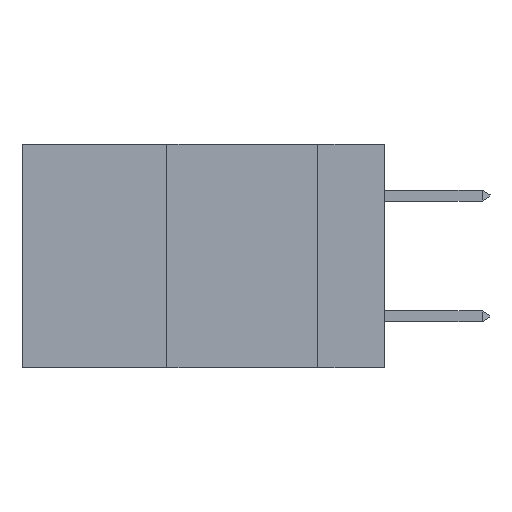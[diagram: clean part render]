
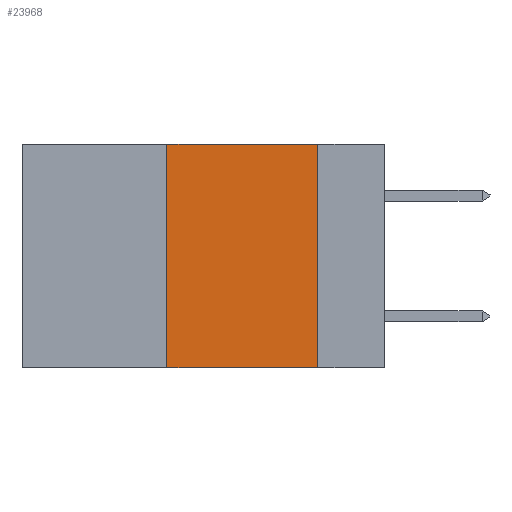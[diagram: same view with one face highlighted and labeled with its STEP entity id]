
A CAD part, left-side view. The second image highlights one B-rep face of the part: STEP entity #23968.
In plain terms, the highlighted planar face has unit normal (-1, 0, 0).
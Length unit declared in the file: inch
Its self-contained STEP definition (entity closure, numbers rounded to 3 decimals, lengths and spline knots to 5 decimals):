
#1269 = CARTESIAN_POINT ( 'NONE',  ( 0., 0.11, 0. ) ) ;
#1663 = EDGE_CURVE ( 'NONE', #42883, #34363, #5095, .T. ) ;
#2012 = CARTESIAN_POINT ( 'NONE',  ( 0., 0.11, 0. ) ) ;
#2697 = VECTOR ( 'NONE', #39720, 39.37008 ) ;
#3630 = DIRECTION ( 'NONE',  ( 0., 0., -1. ) ) ;
#4990 = CARTESIAN_POINT ( 'NONE',  ( 0., 0.11, -0.37 ) ) ;
#5095 = LINE ( 'NONE', #12805, #23792 ) ;
#5523 = VERTEX_POINT ( 'NONE', #38459 ) ;
#6463 = LINE ( 'NONE', #31687, #2697 ) ;
#7240 = PLANE ( 'NONE',  #22509 ) ;
#7541 = DIRECTION ( 'NONE',  ( 1., 0., 0. ) ) ;
#11356 = ORIENTED_EDGE ( 'NONE', *, *, #36620, .F. ) ;
#12805 = CARTESIAN_POINT ( 'NONE',  ( 0., 0.6, 0. ) ) ;
#14676 = FACE_OUTER_BOUND ( 'NONE', #22006, .T. ) ;
#15324 = DIRECTION ( 'NONE',  ( 0., 0., -1. ) ) ;
#18282 = EDGE_CURVE ( 'NONE', #5523, #28503, #6463, .T. ) ;
#18387 = EDGE_CURVE ( 'NONE', #5523, #42883, #27844, .T. ) ;
#19488 = ORIENTED_EDGE ( 'NONE', *, *, #18282, .T. ) ;
#22006 = EDGE_LOOP ( 'NONE', ( #11356, #32466, #23776, #19488 ) ) ;
#22509 = AXIS2_PLACEMENT_3D ( 'NONE', #24111, #7541, #3630 ) ;
#23776 = ORIENTED_EDGE ( 'NONE', *, *, #18387, .F. ) ;
#23792 = VECTOR ( 'NONE', #36936, 39.37008 ) ;
#23968 = ADVANCED_FACE ( 'NONE', ( #14676 ), #7240, .F. ) ;
#24111 = CARTESIAN_POINT ( 'NONE',  ( 0., 0.6, 0. ) ) ;
#25731 = CARTESIAN_POINT ( 'NONE',  ( 0., 0.36, 0. ) ) ;
#27844 = LINE ( 'NONE', #25731, #40106 ) ;
#28503 = VERTEX_POINT ( 'NONE', #4990 ) ;
#29575 = CARTESIAN_POINT ( 'NONE',  ( 0., 0.36, 0. ) ) ;
#31687 = CARTESIAN_POINT ( 'NONE',  ( 0., 0.6, -0.37 ) ) ;
#32466 = ORIENTED_EDGE ( 'NONE', *, *, #1663, .F. ) ;
#34363 = VERTEX_POINT ( 'NONE', #1269 ) ;
#36620 = EDGE_CURVE ( 'NONE', #34363, #28503, #39181, .T. ) ;
#36936 = DIRECTION ( 'NONE',  ( 0., -1., 0. ) ) ;
#38459 = CARTESIAN_POINT ( 'NONE',  ( 0., 0.36, -0.37 ) ) ;
#39181 = LINE ( 'NONE', #2012, #41881 ) ;
#39432 = DIRECTION ( 'NONE',  ( 0., 0., 1. ) ) ;
#39720 = DIRECTION ( 'NONE',  ( 0., -1., 0. ) ) ;
#40106 = VECTOR ( 'NONE', #39432, 39.37008 ) ;
#41881 = VECTOR ( 'NONE', #15324, 39.37008 ) ;
#42883 = VERTEX_POINT ( 'NONE', #29575 ) ;
